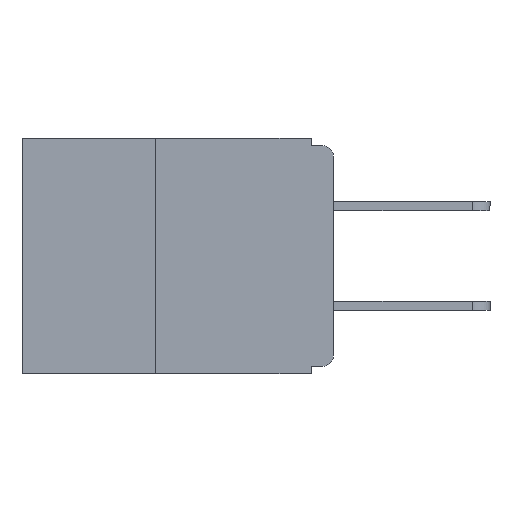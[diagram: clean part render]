
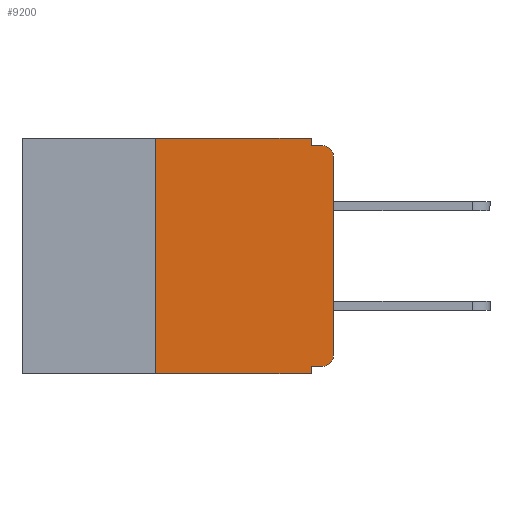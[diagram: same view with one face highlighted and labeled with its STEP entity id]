
A CAD part, left-side view. The second image highlights one B-rep face of the part: STEP entity #9200.
In plain terms, the highlighted planar face has unit normal (-1, 0, 0).
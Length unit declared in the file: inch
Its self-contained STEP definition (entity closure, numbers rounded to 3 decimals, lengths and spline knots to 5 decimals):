
#12 = VECTOR ( 'NONE', #3556, 39.37008 ) ;
#653 = LINE ( 'NONE', #5747, #11422 ) ;
#1350 = CARTESIAN_POINT ( 'NONE',  ( 0., 0.031, -0.33 ) ) ;
#1405 = CARTESIAN_POINT ( 'NONE',  ( 0., 0.437, -0.33 ) ) ;
#1932 = ORIENTED_EDGE ( 'NONE', *, *, #10381, .F. ) ;
#1938 = CARTESIAN_POINT ( 'NONE',  ( 0., 0., -0.32 ) ) ;
#2016 = CARTESIAN_POINT ( 'NONE',  ( 0., 0.015, -0.305 ) ) ;
#2027 = VECTOR ( 'NONE', #8891, 39.37008 ) ;
#2161 = CARTESIAN_POINT ( 'NONE',  ( 0., 0.437, 0. ) ) ;
#2208 = LINE ( 'NONE', #8626, #12972 ) ;
#2305 = VERTEX_POINT ( 'NONE', #9329 ) ;
#2490 = DIRECTION ( 'NONE',  ( 0., 0., 1. ) ) ;
#3010 = EDGE_CURVE ( 'NONE', #8060, #9681, #13278, .T. ) ;
#3087 = DIRECTION ( 'NONE',  ( 0., 0., -1. ) ) ;
#3312 = DIRECTION ( 'NONE',  ( 0., 0., -1. ) ) ;
#3468 = AXIS2_PLACEMENT_3D ( 'NONE', #10629, #4422, #11702 ) ;
#3556 = DIRECTION ( 'NONE',  ( 0., -1., 0. ) ) ;
#3564 = CARTESIAN_POINT ( 'NONE',  ( 0., 0.015, -0.32 ) ) ;
#3697 = ORIENTED_EDGE ( 'NONE', *, *, #8898, .F. ) ;
#3852 = DIRECTION ( 'NONE',  ( -1., 0., 0. ) ) ;
#3952 = DIRECTION ( 'NONE',  ( 0., -1., 0. ) ) ;
#3970 = CARTESIAN_POINT ( 'NONE',  ( 0., 0.015, -0.025 ) ) ;
#4033 = VERTEX_POINT ( 'NONE', #9994 ) ;
#4090 = EDGE_CURVE ( 'NONE', #4033, #12641, #8815, .T. ) ;
#4132 = CARTESIAN_POINT ( 'NONE',  ( 0., 0.015, -0.01 ) ) ;
#4228 = EDGE_CURVE ( 'NONE', #2305, #12641, #653, .T. ) ;
#4422 = DIRECTION ( 'NONE',  ( 1., 0., 0. ) ) ;
#4895 = ORIENTED_EDGE ( 'NONE', *, *, #6239, .T. ) ;
#5370 = CIRCLE ( 'NONE', #10972, 0.015 ) ;
#5747 = CARTESIAN_POINT ( 'NONE',  ( 0., 0., -0.01 ) ) ;
#5962 = FACE_OUTER_BOUND ( 'NONE', #6541, .T. ) ;
#6089 = LINE ( 'NONE', #7024, #8515 ) ;
#6239 = EDGE_CURVE ( 'NONE', #12310, #8258, #5370, .T. ) ;
#6262 = VECTOR ( 'NONE', #10408, 39.37008 ) ;
#6541 = EDGE_LOOP ( 'NONE', ( #12321, #10915, #11103, #11315, #9185, #1932, #11728, #13414, #3697, #4895 ) ) ;
#6719 = CARTESIAN_POINT ( 'NONE',  ( 0., 0.25, -0.33 ) ) ;
#7024 = CARTESIAN_POINT ( 'NONE',  ( 0., 0.031, 0. ) ) ;
#7720 = EDGE_CURVE ( 'NONE', #8258, #4033, #7957, .T. ) ;
#7845 = CARTESIAN_POINT ( 'NONE',  ( 0., 0.25, -0.33 ) ) ;
#7957 = LINE ( 'NONE', #9734, #10372 ) ;
#8060 = VERTEX_POINT ( 'NONE', #6719 ) ;
#8063 = DIRECTION ( 'NONE',  ( 0., 0., -1. ) ) ;
#8073 = CARTESIAN_POINT ( 'NONE',  ( 0., 0., -0.305 ) ) ;
#8258 = VERTEX_POINT ( 'NONE', #8073 ) ;
#8502 = PLANE ( 'NONE',  #3468 ) ;
#8515 = VECTOR ( 'NONE', #8063, 39.37008 ) ;
#8619 = VERTEX_POINT ( 'NONE', #11861 ) ;
#8626 = CARTESIAN_POINT ( 'NONE',  ( 0., 0.031, -0.33 ) ) ;
#8815 = CIRCLE ( 'NONE', #13082, 0.015 ) ;
#8891 = DIRECTION ( 'NONE',  ( 0., 0., 1. ) ) ;
#8898 = EDGE_CURVE ( 'NONE', #12310, #8619, #12341, .T. ) ;
#9185 = ORIENTED_EDGE ( 'NONE', *, *, #10704, .F. ) ;
#9200 = ADVANCED_FACE ( 'NONE', ( #5962 ), #8502, .F. ) ;
#9260 = DIRECTION ( 'NONE',  ( -1., 0., 0. ) ) ;
#9329 = CARTESIAN_POINT ( 'NONE',  ( 0., 0.031, -0.01 ) ) ;
#9387 = CARTESIAN_POINT ( 'NONE',  ( 0., 0.031, 0. ) ) ;
#9681 = VERTEX_POINT ( 'NONE', #1350 ) ;
#9693 = EDGE_CURVE ( 'NONE', #8619, #9681, #2208, .T. ) ;
#9734 = CARTESIAN_POINT ( 'NONE',  ( 0., 0., 0. ) ) ;
#9994 = CARTESIAN_POINT ( 'NONE',  ( 0., 0., -0.025 ) ) ;
#10295 = LINE ( 'NONE', #7845, #2027 ) ;
#10372 = VECTOR ( 'NONE', #2490, 39.37008 ) ;
#10381 = EDGE_CURVE ( 'NONE', #8060, #13012, #10295, .T. ) ;
#10408 = DIRECTION ( 'NONE',  ( 0., -1., 0. ) ) ;
#10629 = CARTESIAN_POINT ( 'NONE',  ( 0., 0.437, 0. ) ) ;
#10704 = EDGE_CURVE ( 'NONE', #13012, #11805, #11345, .T. ) ;
#10712 = DIRECTION ( 'NONE',  ( 0., 0., -1. ) ) ;
#10915 = ORIENTED_EDGE ( 'NONE', *, *, #4090, .T. ) ;
#10972 = AXIS2_PLACEMENT_3D ( 'NONE', #2016, #9260, #3087 ) ;
#11103 = ORIENTED_EDGE ( 'NONE', *, *, #4228, .F. ) ;
#11315 = ORIENTED_EDGE ( 'NONE', *, *, #12518, .F. ) ;
#11345 = LINE ( 'NONE', #2161, #6262 ) ;
#11422 = VECTOR ( 'NONE', #3952, 39.37008 ) ;
#11702 = DIRECTION ( 'NONE',  ( 0., 0., -1. ) ) ;
#11728 = ORIENTED_EDGE ( 'NONE', *, *, #3010, .T. ) ;
#11805 = VERTEX_POINT ( 'NONE', #9387 ) ;
#11861 = CARTESIAN_POINT ( 'NONE',  ( 0., 0.031, -0.32 ) ) ;
#12006 = VECTOR ( 'NONE', #13369, 39.37008 ) ;
#12074 = CARTESIAN_POINT ( 'NONE',  ( 0., 0.25, 0. ) ) ;
#12310 = VERTEX_POINT ( 'NONE', #3564 ) ;
#12321 = ORIENTED_EDGE ( 'NONE', *, *, #7720, .T. ) ;
#12341 = LINE ( 'NONE', #1938, #12006 ) ;
#12518 = EDGE_CURVE ( 'NONE', #11805, #2305, #6089, .T. ) ;
#12641 = VERTEX_POINT ( 'NONE', #4132 ) ;
#12972 = VECTOR ( 'NONE', #10712, 39.37008 ) ;
#13012 = VERTEX_POINT ( 'NONE', #12074 ) ;
#13082 = AXIS2_PLACEMENT_3D ( 'NONE', #3970, #3852, #3312 ) ;
#13278 = LINE ( 'NONE', #1405, #12 ) ;
#13369 = DIRECTION ( 'NONE',  ( 0., 1., 0. ) ) ;
#13414 = ORIENTED_EDGE ( 'NONE', *, *, #9693, .F. ) ;
